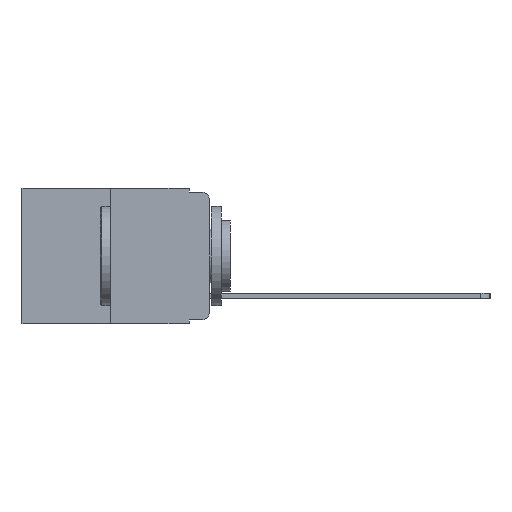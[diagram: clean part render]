
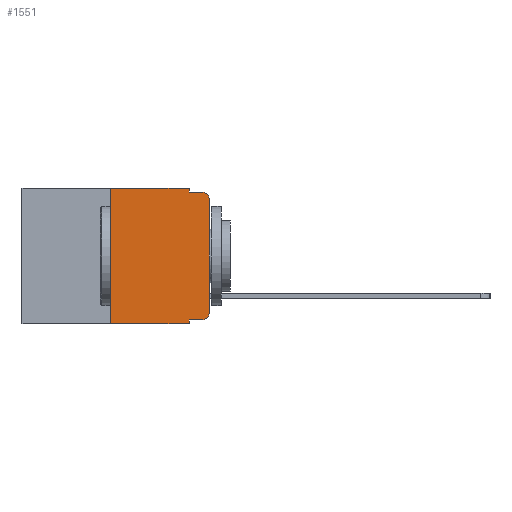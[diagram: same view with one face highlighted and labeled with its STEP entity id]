
A CAD part, left-side view. The second image highlights one B-rep face of the part: STEP entity #1551.
In plain terms, the highlighted planar face has unit normal (-1, 0, 0).
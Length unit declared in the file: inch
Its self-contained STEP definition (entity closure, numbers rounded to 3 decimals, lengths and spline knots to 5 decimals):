
#29 = LINE ( 'NONE', #13240, #9325 ) ;
#80 = CARTESIAN_POINT ( 'NONE',  ( 0., 0., -0.03 ) ) ;
#229 = CARTESIAN_POINT ( 'NONE',  ( 0., 0.051, -0.333 ) ) ;
#966 = VERTEX_POINT ( 'NONE', #4409 ) ;
#1089 = ORIENTED_EDGE ( 'NONE', *, *, #12125, .F. ) ;
#1382 = DIRECTION ( 'NONE',  ( -1., 0., 0. ) ) ;
#1550 = EDGE_CURVE ( 'NONE', #2533, #966, #2416, .T. ) ;
#1551 = ADVANCED_FACE ( 'NONE', ( #11193 ), #7010, .F. ) ;
#1778 = EDGE_CURVE ( 'NONE', #7634, #9724, #6412, .T. ) ;
#1931 = EDGE_LOOP ( 'NONE', ( #4076, #7260, #10155, #1089, #13271, #7969, #10809, #8665, #11474, #12119 ) ) ;
#2306 = CARTESIAN_POINT ( 'NONE',  ( 0., 0.02, -0.01 ) ) ;
#2323 = CIRCLE ( 'NONE', #12973, 0.02 ) ;
#2416 = LINE ( 'NONE', #8814, #13648 ) ;
#2533 = VERTEX_POINT ( 'NONE', #14748 ) ;
#2571 = LINE ( 'NONE', #3150, #8529 ) ;
#3069 = VERTEX_POINT ( 'NONE', #11113 ) ;
#3150 = CARTESIAN_POINT ( 'NONE',  ( 0., 0.25, 0. ) ) ;
#3192 = CARTESIAN_POINT ( 'NONE',  ( 0., 0.051, 0. ) ) ;
#3598 = VERTEX_POINT ( 'NONE', #80 ) ;
#3769 = CARTESIAN_POINT ( 'NONE',  ( 0., 0., 0. ) ) ;
#4076 = ORIENTED_EDGE ( 'NONE', *, *, #14246, .T. ) ;
#4409 = CARTESIAN_POINT ( 'NONE',  ( 0., 0.051, -0.343 ) ) ;
#4455 = AXIS2_PLACEMENT_3D ( 'NONE', #8604, #1382, #9661 ) ;
#4974 = CARTESIAN_POINT ( 'NONE',  ( 0., 0.25, 0. ) ) ;
#5194 = VERTEX_POINT ( 'NONE', #13410 ) ;
#6412 = LINE ( 'NONE', #8212, #11520 ) ;
#6423 = LINE ( 'NONE', #3769, #11844 ) ;
#6503 = CARTESIAN_POINT ( 'NONE',  ( 0., 0.02, -0.03 ) ) ;
#6599 = LINE ( 'NONE', #6951, #14809 ) ;
#6821 = DIRECTION ( 'NONE',  ( 0., 0., -1. ) ) ;
#6909 = VERTEX_POINT ( 'NONE', #12000 ) ;
#6951 = CARTESIAN_POINT ( 'NONE',  ( 0., 0.051, 0. ) ) ;
#7010 = PLANE ( 'NONE',  #12804 ) ;
#7260 = ORIENTED_EDGE ( 'NONE', *, *, #13537, .T. ) ;
#7333 = LINE ( 'NONE', #14672, #12693 ) ;
#7456 = VECTOR ( 'NONE', #8772, 39.37008 ) ;
#7479 = DIRECTION ( 'NONE',  ( 1., 0., 0. ) ) ;
#7634 = VERTEX_POINT ( 'NONE', #4974 ) ;
#7658 = DIRECTION ( 'NONE',  ( 0., 0., -1. ) ) ;
#7665 = CARTESIAN_POINT ( 'NONE',  ( 0., 0.051, 0. ) ) ;
#7820 = LINE ( 'NONE', #7665, #7456 ) ;
#7944 = CARTESIAN_POINT ( 'NONE',  ( 0., 0.473, 0. ) ) ;
#7969 = ORIENTED_EDGE ( 'NONE', *, *, #11436, .F. ) ;
#8101 = DIRECTION ( 'NONE',  ( 0., -1., 0. ) ) ;
#8212 = CARTESIAN_POINT ( 'NONE',  ( 0., 0.473, 0. ) ) ;
#8529 = VECTOR ( 'NONE', #9017, 39.37008 ) ;
#8604 = CARTESIAN_POINT ( 'NONE',  ( 0., 0.02, -0.313 ) ) ;
#8665 = ORIENTED_EDGE ( 'NONE', *, *, #10725, .F. ) ;
#8772 = DIRECTION ( 'NONE',  ( 0., 0., -1. ) ) ;
#8814 = CARTESIAN_POINT ( 'NONE',  ( 0., 0.473, -0.343 ) ) ;
#9017 = DIRECTION ( 'NONE',  ( 0., 0., 1. ) ) ;
#9106 = VERTEX_POINT ( 'NONE', #2306 ) ;
#9311 = EDGE_CURVE ( 'NONE', #5194, #6909, #11287, .T. ) ;
#9325 = VECTOR ( 'NONE', #14301, 39.37008 ) ;
#9556 = DIRECTION ( 'NONE',  ( 0., 0., 1. ) ) ;
#9661 = DIRECTION ( 'NONE',  ( 0., 0., -1. ) ) ;
#9724 = VERTEX_POINT ( 'NONE', #3192 ) ;
#10028 = EDGE_CURVE ( 'NONE', #13551, #5194, #7333, .T. ) ;
#10155 = ORIENTED_EDGE ( 'NONE', *, *, #12848, .F. ) ;
#10484 = DIRECTION ( 'NONE',  ( 0., -1., 0. ) ) ;
#10725 = EDGE_CURVE ( 'NONE', #13551, #966, #6599, .T. ) ;
#10809 = ORIENTED_EDGE ( 'NONE', *, *, #1550, .T. ) ;
#11113 = CARTESIAN_POINT ( 'NONE',  ( 0., 0.051, -0.01 ) ) ;
#11193 = FACE_OUTER_BOUND ( 'NONE', #1931, .T. ) ;
#11245 = DIRECTION ( 'NONE',  ( 0., 0., -1. ) ) ;
#11287 = CIRCLE ( 'NONE', #4455, 0.02 ) ;
#11293 = DIRECTION ( 'NONE',  ( 0., -1., 0. ) ) ;
#11436 = EDGE_CURVE ( 'NONE', #2533, #7634, #2571, .T. ) ;
#11474 = ORIENTED_EDGE ( 'NONE', *, *, #10028, .T. ) ;
#11520 = VECTOR ( 'NONE', #8101, 39.37008 ) ;
#11844 = VECTOR ( 'NONE', #9556, 39.37008 ) ;
#12000 = CARTESIAN_POINT ( 'NONE',  ( 0., 0., -0.313 ) ) ;
#12119 = ORIENTED_EDGE ( 'NONE', *, *, #9311, .T. ) ;
#12125 = EDGE_CURVE ( 'NONE', #9724, #3069, #7820, .T. ) ;
#12693 = VECTOR ( 'NONE', #10484, 39.37008 ) ;
#12804 = AXIS2_PLACEMENT_3D ( 'NONE', #7944, #7479, #6821 ) ;
#12848 = EDGE_CURVE ( 'NONE', #3069, #9106, #29, .T. ) ;
#12973 = AXIS2_PLACEMENT_3D ( 'NONE', #6503, #14005, #7658 ) ;
#13240 = CARTESIAN_POINT ( 'NONE',  ( 0., 0.051, -0.01 ) ) ;
#13271 = ORIENTED_EDGE ( 'NONE', *, *, #1778, .F. ) ;
#13410 = CARTESIAN_POINT ( 'NONE',  ( 0., 0.02, -0.333 ) ) ;
#13537 = EDGE_CURVE ( 'NONE', #3598, #9106, #2323, .T. ) ;
#13551 = VERTEX_POINT ( 'NONE', #229 ) ;
#13648 = VECTOR ( 'NONE', #11293, 39.37008 ) ;
#14005 = DIRECTION ( 'NONE',  ( -1., 0., 0. ) ) ;
#14246 = EDGE_CURVE ( 'NONE', #6909, #3598, #6423, .T. ) ;
#14301 = DIRECTION ( 'NONE',  ( 0., -1., 0. ) ) ;
#14672 = CARTESIAN_POINT ( 'NONE',  ( 0., 0.051, -0.333 ) ) ;
#14748 = CARTESIAN_POINT ( 'NONE',  ( 0., 0.25, -0.343 ) ) ;
#14809 = VECTOR ( 'NONE', #11245, 39.37008 ) ;
